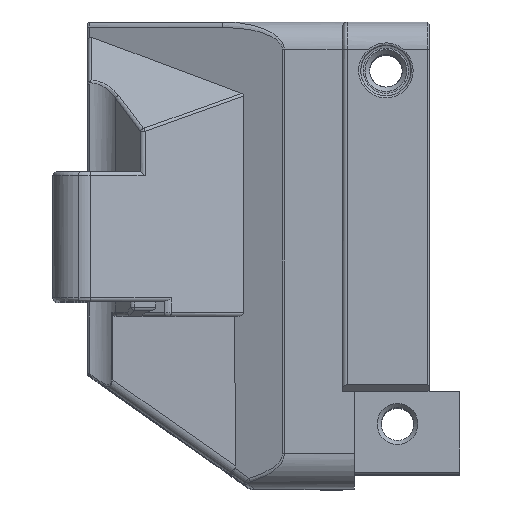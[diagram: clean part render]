
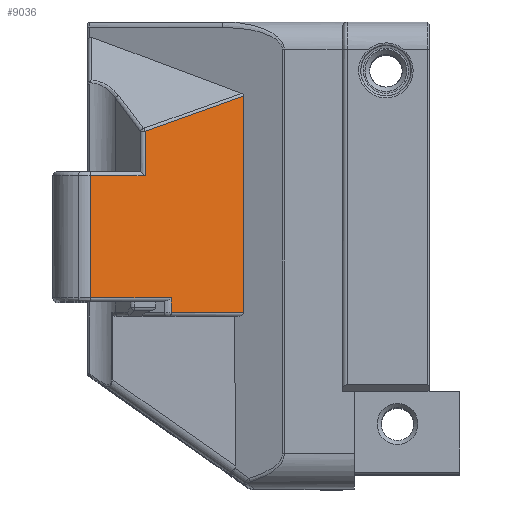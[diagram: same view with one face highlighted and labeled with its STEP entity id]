
A CAD part, top view. The second image highlights one B-rep face of the part: STEP entity #9036.
In plain terms, the highlighted planar face has unit normal (0.336, 0, 0.942).
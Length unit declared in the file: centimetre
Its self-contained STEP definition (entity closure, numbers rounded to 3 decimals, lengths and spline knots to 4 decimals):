
#447=PLANE($,#9981);
#1079=LINE($,#17340,#1812);
#1080=LINE($,#17350,#1813);
#1081=LINE($,#17352,#1814);
#1082=LINE($,#17355,#1815);
#1083=LINE($,#17359,#1816);
#1145=LINE($,#18202,#1878);
#1146=LINE($,#18205,#1879);
#1147=LINE($,#18206,#1880);
#1812=VECTOR($,#12231,0.2905);
#1813=VECTOR($,#12234,1.6989);
#1814=VECTOR($,#12237,2.4231);
#1815=VECTOR($,#12240,1.1462);
#1816=VECTOR($,#12245,0.8825);
#1878=VECTOR($,#12497,1.5242);
#1879=VECTOR($,#12500,4.2946);
#1880=VECTOR($,#12501,2.1912);
#2619=FACE_OUTER_BOUND($,#3212,.T.);
#3212=EDGE_LOOP($,(#8219,#8220,#8221,#8222,#8223,#8224,#8225,#8226));
#4372=VERTEX_POINT($,#16638);
#4377=VERTEX_POINT($,#16649);
#4445=VERTEX_POINT($,#17334);
#4446=VERTEX_POINT($,#17339);
#4447=VERTEX_POINT($,#17354);
#4448=VERTEX_POINT($,#17358);
#4520=VERTEX_POINT($,#18200);
#4521=VERTEX_POINT($,#18204);
#5653=EDGE_CURVE($,#4445,#4446,#1079,.T.);
#5655=EDGE_CURVE($,#4446,#4372,#1080,.T.);
#5656=EDGE_CURVE($,#4372,#4377,#1081,.T.);
#5657=EDGE_CURVE($,#4377,#4447,#1082,.T.);
#5659=EDGE_CURVE($,#4447,#4448,#1083,.T.);
#5783=EDGE_CURVE($,#4520,#4445,#1145,.T.);
#5784=EDGE_CURVE($,#4521,#4520,#1146,.T.);
#5785=EDGE_CURVE($,#4448,#4521,#1147,.T.);
#8219=ORIENTED_EDGE($,*,*,#5784,.F.);
#8220=ORIENTED_EDGE($,*,*,#5785,.F.);
#8221=ORIENTED_EDGE($,*,*,#5659,.F.);
#8222=ORIENTED_EDGE($,*,*,#5657,.F.);
#8223=ORIENTED_EDGE($,*,*,#5656,.F.);
#8224=ORIENTED_EDGE($,*,*,#5655,.F.);
#8225=ORIENTED_EDGE($,*,*,#5653,.F.);
#8226=ORIENTED_EDGE($,*,*,#5783,.F.);
#9036=ADVANCED_FACE($,(#2619),#447,.T.);
#9981=AXIS2_PLACEMENT_3D($,#18203,#12498,#12499);
#12231=DIRECTION($,(0.,1.,0.));
#12234=DIRECTION($,(-0.942,0.,0.336));
#12237=DIRECTION($,(0.,1.,0.));
#12240=DIRECTION($,(0.942,0.,-0.336));
#12245=DIRECTION($,(0.,1.,0.));
#12497=DIRECTION($,(-0.942,0.,0.336));
#12498=DIRECTION('center_axis',(0.336,0.,
0.942));
#12499=DIRECTION('ref_axis',(0.942,0.,-0.336));
#12500=DIRECTION($,(0.,-1.,0.));
#12501=DIRECTION($,(0.893,0.319,-0.319));
#16638=CARTESIAN_POINT('',(-24.5909,2.4372,12.7451));
#16649=CARTESIAN_POINT('',(-24.5909,4.8603,12.7451));
#17334=CARTESIAN_POINT('',(-22.9909,2.1467,12.1737));
#17339=CARTESIAN_POINT('',(-22.9909,2.4372,12.1737));
#17340=CARTESIAN_POINT($,(-22.9909,4.6523,12.1737));
#17350=CARTESIAN_POINT($,(-23.4879,2.4372,12.3512));
#17352=CARTESIAN_POINT($,(-24.5909,4.9403,12.7451));
#17354=CARTESIAN_POINT('',(-23.5114,4.8603,12.3595));
#17355=CARTESIAN_POINT($,(-24.1436,4.8603,12.5854));
#17358=CARTESIAN_POINT('',(-23.5114,5.7428,12.3595));
#17359=CARTESIAN_POINT($,(-23.5114,4.5331,12.3595));
#18200=CARTESIAN_POINT('',(-21.5555,2.1467,11.661));
#18202=CARTESIAN_POINT($,(-21.8472,2.1467,11.7652));
#18203=CARTESIAN_POINT('Origin',(-23.8523,4.1259,12.4813));
#18204=CARTESIAN_POINT('',(-21.5555,6.4413,11.661));
#18205=CARTESIAN_POINT($,(-21.5555,1.3862,11.661));
#18206=CARTESIAN_POINT($,(-23.9117,5.5998,12.5025));
